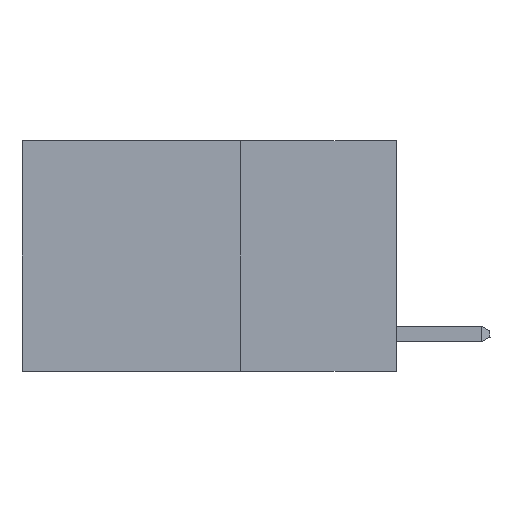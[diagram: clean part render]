
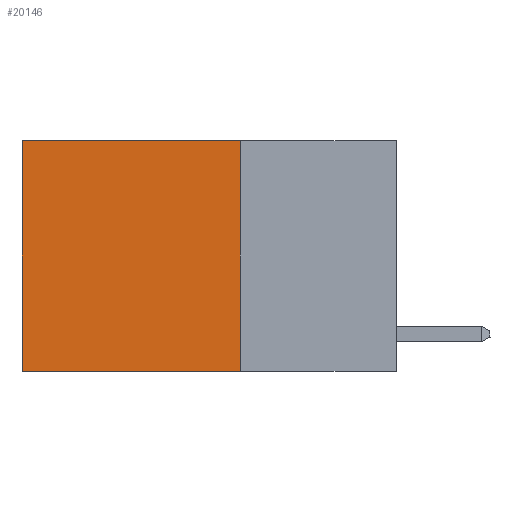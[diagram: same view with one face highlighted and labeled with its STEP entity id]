
A CAD part, left-side view. The second image highlights one B-rep face of the part: STEP entity #20146.
In plain terms, the highlighted planar face has unit normal (-1, 0, 0).
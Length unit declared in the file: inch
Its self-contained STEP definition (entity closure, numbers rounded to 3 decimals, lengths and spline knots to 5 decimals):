
#191 = DIRECTION ( 'NONE',  ( 1., 0., 0. ) ) ;
#1381 = CARTESIAN_POINT ( 'NONE',  ( 0.2625, 0.25, -0.37 ) ) ;
#3387 = CARTESIAN_POINT ( 'NONE',  ( 0.2625, 0.6, -0.37 ) ) ;
#4488 = CARTESIAN_POINT ( 'NONE',  ( 0.2625, 0.25, -0.37 ) ) ;
#6365 = LINE ( 'NONE', #8799, #21954 ) ;
#8373 = LINE ( 'NONE', #14148, #20122 ) ;
#8446 = LINE ( 'NONE', #22786, #17669 ) ;
#8799 = CARTESIAN_POINT ( 'NONE',  ( 0.2625, 0.6, 0. ) ) ;
#8926 = EDGE_LOOP ( 'NONE', ( #16407, #22566, #22091, #16989 ) ) ;
#10545 = DIRECTION ( 'NONE',  ( 0., 0., -1. ) ) ;
#10786 = PLANE ( 'NONE',  #22110 ) ;
#10842 = EDGE_CURVE ( 'NONE', #26398, #15015, #8373, .T. ) ;
#11105 = VERTEX_POINT ( 'NONE', #1381 ) ;
#12551 = DIRECTION ( 'NONE',  ( 0., 1., 0. ) ) ;
#13197 = CARTESIAN_POINT ( 'NONE',  ( 0.2625, 0.6, 0. ) ) ;
#14148 = CARTESIAN_POINT ( 'NONE',  ( 0.2625, 0.25, 0. ) ) ;
#15015 = VERTEX_POINT ( 'NONE', #13197 ) ;
#16407 = ORIENTED_EDGE ( 'NONE', *, *, #25265, .T. ) ;
#16551 = DIRECTION ( 'NONE',  ( 0., 0., -1. ) ) ;
#16569 = LINE ( 'NONE', #4488, #19821 ) ;
#16989 = ORIENTED_EDGE ( 'NONE', *, *, #10842, .T. ) ;
#17669 = VECTOR ( 'NONE', #20780, 39.37008 ) ;
#18180 = VERTEX_POINT ( 'NONE', #3387 ) ;
#19821 = VECTOR ( 'NONE', #12551, 39.37008 ) ;
#20122 = VECTOR ( 'NONE', #22314, 39.37008 ) ;
#20146 = ADVANCED_FACE ( 'NONE', ( #20570 ), #10786, .F. ) ;
#20203 = CARTESIAN_POINT ( 'NONE',  ( 0.2625, 0.25, 0. ) ) ;
#20570 = FACE_OUTER_BOUND ( 'NONE', #8926, .T. ) ;
#20780 = DIRECTION ( 'NONE',  ( 0., 0., -1. ) ) ;
#21954 = VECTOR ( 'NONE', #10545, 39.37008 ) ;
#22091 = ORIENTED_EDGE ( 'NONE', *, *, #23071, .F. ) ;
#22110 = AXIS2_PLACEMENT_3D ( 'NONE', #22981, #191, #16551 ) ;
#22314 = DIRECTION ( 'NONE',  ( 0., 1., 0. ) ) ;
#22566 = ORIENTED_EDGE ( 'NONE', *, *, #25240, .F. ) ;
#22786 = CARTESIAN_POINT ( 'NONE',  ( 0.2625, 0.25, 0. ) ) ;
#22981 = CARTESIAN_POINT ( 'NONE',  ( 0.2625, 0.25, 0. ) ) ;
#23071 = EDGE_CURVE ( 'NONE', #26398, #11105, #8446, .T. ) ;
#25240 = EDGE_CURVE ( 'NONE', #11105, #18180, #16569, .T. ) ;
#25265 = EDGE_CURVE ( 'NONE', #15015, #18180, #6365, .T. ) ;
#26398 = VERTEX_POINT ( 'NONE', #20203 ) ;
